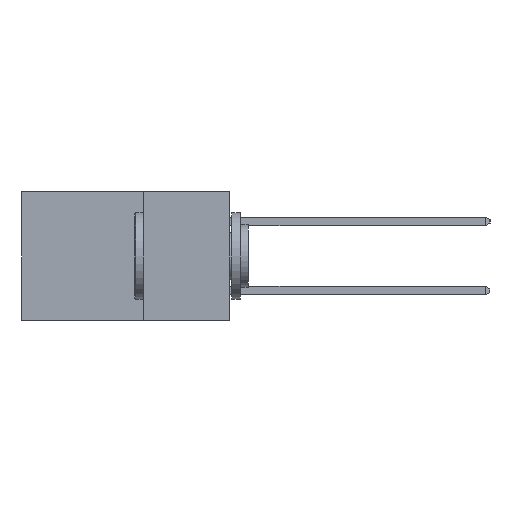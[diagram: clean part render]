
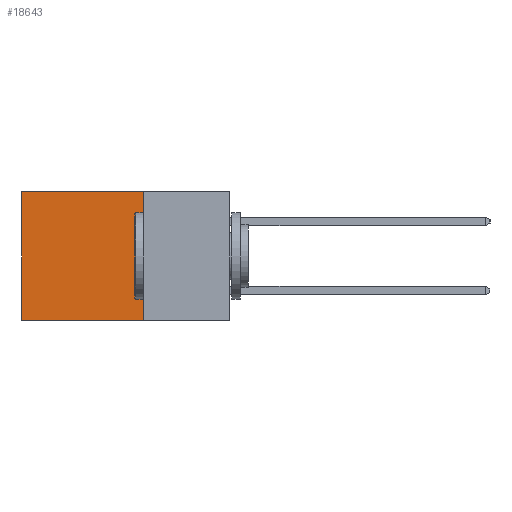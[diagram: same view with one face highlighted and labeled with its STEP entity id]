
A CAD part, left-side view. The second image highlights one B-rep face of the part: STEP entity #18643.
In plain terms, the highlighted planar face has unit normal (-1, 0, 0).
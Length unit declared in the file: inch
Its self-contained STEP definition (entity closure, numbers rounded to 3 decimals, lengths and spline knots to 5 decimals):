
#1307 = CARTESIAN_POINT ( 'NONE',  ( 0.2615, 0.25, -0.37 ) ) ;
#2077 = FACE_OUTER_BOUND ( 'NONE', #5967, .T. ) ;
#2802 = DIRECTION ( 'NONE',  ( 0., 0., -1. ) ) ;
#3148 = DIRECTION ( 'NONE',  ( 0., 1., 0. ) ) ;
#3461 = ORIENTED_EDGE ( 'NONE', *, *, #17852, .F. ) ;
#3732 = VERTEX_POINT ( 'NONE', #13294 ) ;
#4048 = CARTESIAN_POINT ( 'NONE',  ( 0.2615, 0.25, 0. ) ) ;
#4467 = VERTEX_POINT ( 'NONE', #16480 ) ;
#4667 = LINE ( 'NONE', #1307, #13544 ) ;
#5967 = EDGE_LOOP ( 'NONE', ( #11568, #3461, #13942, #18014 ) ) ;
#6674 = VERTEX_POINT ( 'NONE', #8020 ) ;
#6960 = PLANE ( 'NONE',  #11157 ) ;
#7117 = CARTESIAN_POINT ( 'NONE',  ( 0.2615, 0.25, 0. ) ) ;
#8020 = CARTESIAN_POINT ( 'NONE',  ( 0.2615, 0.6, -0.37 ) ) ;
#8132 = EDGE_CURVE ( 'NONE', #4467, #6674, #22047, .T. ) ;
#8496 = LINE ( 'NONE', #4048, #22450 ) ;
#8737 = DIRECTION ( 'NONE',  ( 0., 0., -1. ) ) ;
#9985 = CARTESIAN_POINT ( 'NONE',  ( 0.2615, 0.6, -0.37 ) ) ;
#11139 = VECTOR ( 'NONE', #2802, 39.37008 ) ;
#11157 = AXIS2_PLACEMENT_3D ( 'NONE', #17548, #19280, #8737 ) ;
#11568 = ORIENTED_EDGE ( 'NONE', *, *, #8132, .T. ) ;
#11599 = VERTEX_POINT ( 'NONE', #7117 ) ;
#13294 = CARTESIAN_POINT ( 'NONE',  ( 0.2615, 0.25, -0.37 ) ) ;
#13544 = VECTOR ( 'NONE', #3148, 39.37008 ) ;
#13942 = ORIENTED_EDGE ( 'NONE', *, *, #16439, .F. ) ;
#14661 = DIRECTION ( 'NONE',  ( 0., 1., 0. ) ) ;
#15822 = LINE ( 'NONE', #22119, #11139 ) ;
#16439 = EDGE_CURVE ( 'NONE', #11599, #3732, #15822, .T. ) ;
#16480 = CARTESIAN_POINT ( 'NONE',  ( 0.2615, 0.6, 0. ) ) ;
#17485 = VECTOR ( 'NONE', #20490, 39.37008 ) ;
#17548 = CARTESIAN_POINT ( 'NONE',  ( 0.2615, 0.25, -0.37 ) ) ;
#17852 = EDGE_CURVE ( 'NONE', #3732, #6674, #4667, .T. ) ;
#18014 = ORIENTED_EDGE ( 'NONE', *, *, #18976, .T. ) ;
#18643 = ADVANCED_FACE ( 'NONE', ( #2077 ), #6960, .F. ) ;
#18976 = EDGE_CURVE ( 'NONE', #11599, #4467, #8496, .T. ) ;
#19280 = DIRECTION ( 'NONE',  ( 1., 0., 0. ) ) ;
#20490 = DIRECTION ( 'NONE',  ( 0., 0., -1. ) ) ;
#22047 = LINE ( 'NONE', #9985, #17485 ) ;
#22119 = CARTESIAN_POINT ( 'NONE',  ( 0.2615, 0.25, -0.37 ) ) ;
#22450 = VECTOR ( 'NONE', #14661, 39.37008 ) ;
